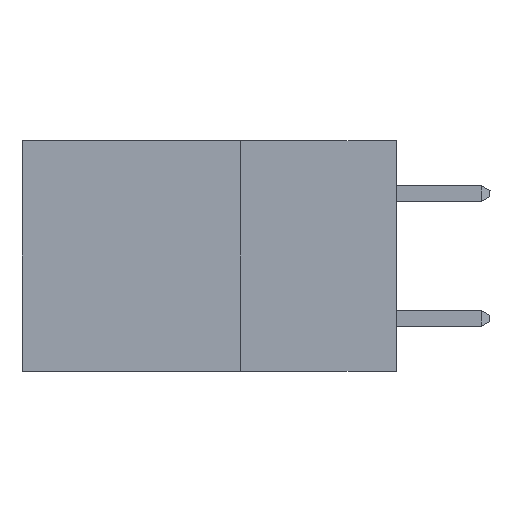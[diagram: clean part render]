
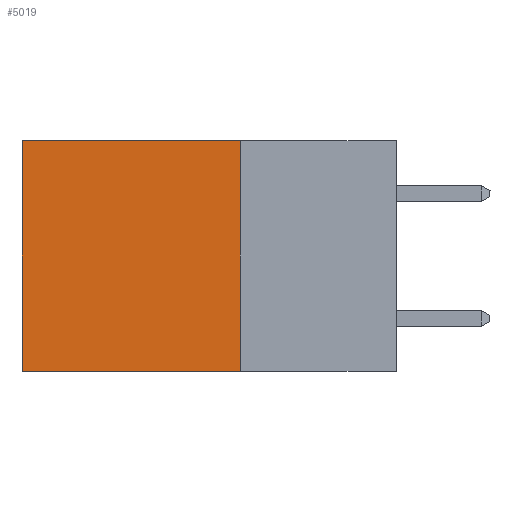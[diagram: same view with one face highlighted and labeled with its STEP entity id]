
A CAD part, left-side view. The second image highlights one B-rep face of the part: STEP entity #5019.
In plain terms, the highlighted planar face has unit normal (-1, 0, 0).
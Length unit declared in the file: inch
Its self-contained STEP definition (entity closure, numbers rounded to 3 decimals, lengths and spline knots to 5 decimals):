
#21 = EDGE_CURVE ( 'NONE', #4041, #5052, #8781, .T. ) ;
#30 = AXIS2_PLACEMENT_3D ( 'NONE', #1412, #2113, #7165 ) ;
#729 = EDGE_CURVE ( 'NONE', #5052, #3608, #2705, .T. ) ;
#853 = VECTOR ( 'NONE', #4229, 39.37008 ) ;
#856 = EDGE_CURVE ( 'NONE', #6218, #3608, #2594, .T. ) ;
#1412 = CARTESIAN_POINT ( 'NONE',  ( 0.298, 0.25, 0. ) ) ;
#1532 = DIRECTION ( 'NONE',  ( 0., 0., -1. ) ) ;
#2041 = CARTESIAN_POINT ( 'NONE',  ( 0.298, 0.25, 0. ) ) ;
#2113 = DIRECTION ( 'NONE',  ( 1., 0., 0. ) ) ;
#2594 = LINE ( 'NONE', #6104, #6233 ) ;
#2705 = LINE ( 'NONE', #5990, #853 ) ;
#3356 = DIRECTION ( 'NONE',  ( 0., 1., 0. ) ) ;
#3507 = CARTESIAN_POINT ( 'NONE',  ( 0.298, 0.25, 0. ) ) ;
#3608 = VERTEX_POINT ( 'NONE', #8112 ) ;
#3998 = VECTOR ( 'NONE', #1532, 39.37008 ) ;
#4041 = VERTEX_POINT ( 'NONE', #2041 ) ;
#4229 = DIRECTION ( 'NONE',  ( 0., 0., -1. ) ) ;
#4531 = ORIENTED_EDGE ( 'NONE', *, *, #856, .F. ) ;
#4574 = DIRECTION ( 'NONE',  ( 0., 1., 0. ) ) ;
#5019 = ADVANCED_FACE ( 'NONE', ( #6493 ), #6432, .F. ) ;
#5052 = VERTEX_POINT ( 'NONE', #5752 ) ;
#5462 = LINE ( 'NONE', #5840, #3998 ) ;
#5752 = CARTESIAN_POINT ( 'NONE',  ( 0.298, 0.6, 0. ) ) ;
#5840 = CARTESIAN_POINT ( 'NONE',  ( 0.298, 0.25, 0. ) ) ;
#5990 = CARTESIAN_POINT ( 'NONE',  ( 0.298, 0.6, 0. ) ) ;
#6104 = CARTESIAN_POINT ( 'NONE',  ( 0.298, 0.25, -0.37 ) ) ;
#6218 = VERTEX_POINT ( 'NONE', #6255 ) ;
#6233 = VECTOR ( 'NONE', #4574, 39.37008 ) ;
#6255 = CARTESIAN_POINT ( 'NONE',  ( 0.298, 0.25, -0.37 ) ) ;
#6432 = PLANE ( 'NONE',  #30 ) ;
#6493 = FACE_OUTER_BOUND ( 'NONE', #7732, .T. ) ;
#6852 = VECTOR ( 'NONE', #3356, 39.37008 ) ;
#7144 = ORIENTED_EDGE ( 'NONE', *, *, #729, .T. ) ;
#7165 = DIRECTION ( 'NONE',  ( 0., 0., -1. ) ) ;
#7586 = ORIENTED_EDGE ( 'NONE', *, *, #21, .T. ) ;
#7732 = EDGE_LOOP ( 'NONE', ( #7144, #4531, #8113, #7586 ) ) ;
#8112 = CARTESIAN_POINT ( 'NONE',  ( 0.298, 0.6, -0.37 ) ) ;
#8113 = ORIENTED_EDGE ( 'NONE', *, *, #8357, .F. ) ;
#8357 = EDGE_CURVE ( 'NONE', #4041, #6218, #5462, .T. ) ;
#8781 = LINE ( 'NONE', #3507, #6852 ) ;
